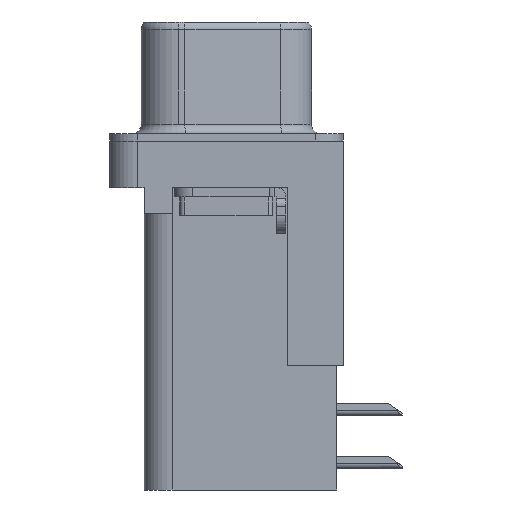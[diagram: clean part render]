
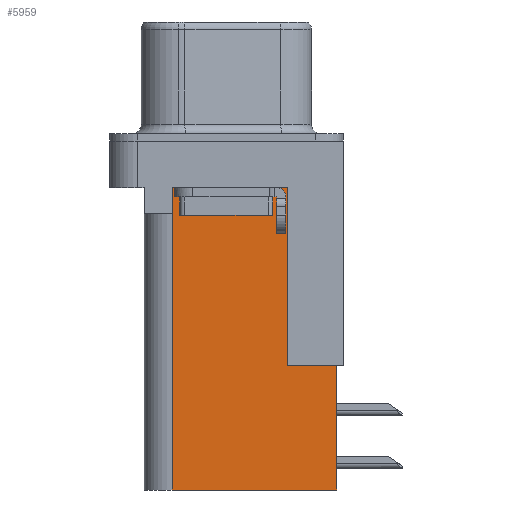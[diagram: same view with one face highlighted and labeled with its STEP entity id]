
A CAD part, left-side view. The second image highlights one B-rep face of the part: STEP entity #5959.
In plain terms, the highlighted planar face has unit normal (-1, 0, 0).
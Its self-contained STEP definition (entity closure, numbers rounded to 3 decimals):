
#126 = CARTESIAN_POINT ( 'NONE',  ( 3.765, -5.925, -2. ) ) ;
#256 = VECTOR ( 'NONE', #9642, 1000. ) ;
#456 = LINE ( 'NONE', #14605, #256 ) ;
#901 = CARTESIAN_POINT ( 'NONE',  ( 3.765, 2.895, -3.9 ) ) ;
#952 = VECTOR ( 'NONE', #4581, 1000. ) ;
#986 = DIRECTION ( 'NONE',  ( 0., 1., 0. ) ) ;
#1053 = LINE ( 'NONE', #12186, #952 ) ;
#1066 = CARTESIAN_POINT ( 'NONE',  ( 3.765, -6.295, -12.05 ) ) ;
#1239 = ORIENTED_EDGE ( 'NONE', *, *, #4993, .F. ) ;
#1700 = EDGE_LOOP ( 'NONE', ( #2459, #14002, #16082, #8216, #1239, #6621, #13790, #6805 ) ) ;
#1952 = LINE ( 'NONE', #14886, #2027 ) ;
#2027 = VECTOR ( 'NONE', #6052, 1000. ) ;
#2459 = ORIENTED_EDGE ( 'NONE', *, *, #7553, .T. ) ;
#2877 = EDGE_CURVE ( 'NONE', #8169, #6811, #7024, .T. ) ;
#3141 = DIRECTION ( 'NONE',  ( 1., 0., 0. ) ) ;
#3420 = CARTESIAN_POINT ( 'NONE',  ( 3.765, 2.925, -18.76 ) ) ;
#3614 = EDGE_CURVE ( 'NONE', #8169, #12137, #4800, .T. ) ;
#4581 = DIRECTION ( 'NONE',  ( 0., 1., 0. ) ) ;
#4800 = LINE ( 'NONE', #1066, #4847 ) ;
#4823 = CARTESIAN_POINT ( 'NONE',  ( 3.765, -3.295, -12.05 ) ) ;
#4847 = VECTOR ( 'NONE', #986, 1000. ) ;
#4993 = EDGE_CURVE ( 'NONE', #6811, #10145, #1053, .T. ) ;
#5348 = VECTOR ( 'NONE', #11344, 1000. ) ;
#5446 = LINE ( 'NONE', #901, #5348 ) ;
#5807 = DIRECTION ( 'NONE',  ( 0., 0., -1. ) ) ;
#5915 = VERTEX_POINT ( 'NONE', #12003 ) ;
#5959 = ADVANCED_FACE ( 'NONE', ( #14445 ), #8398, .F. ) ;
#6052 = DIRECTION ( 'NONE',  ( 0., 1., 0. ) ) ;
#6077 = VERTEX_POINT ( 'NONE', #8673 ) ;
#6144 = CARTESIAN_POINT ( 'NONE',  ( 3.765, -5.925, -12.05 ) ) ;
#6621 = ORIENTED_EDGE ( 'NONE', *, *, #2877, .F. ) ;
#6805 = ORIENTED_EDGE ( 'NONE', *, *, #13910, .T. ) ;
#6811 = VERTEX_POINT ( 'NONE', #9026 ) ;
#7024 = LINE ( 'NONE', #126, #7094 ) ;
#7047 = CARTESIAN_POINT ( 'NONE',  ( 3.765, -3.295, -18.76 ) ) ;
#7094 = VECTOR ( 'NONE', #5807, 1000. ) ;
#7225 = VECTOR ( 'NONE', #8335, 1000. ) ;
#7266 = LINE ( 'NONE', #14501, #7225 ) ;
#7553 = EDGE_CURVE ( 'NONE', #6077, #5915, #9296, .T. ) ;
#7623 = VERTEX_POINT ( 'NONE', #12732 ) ;
#7832 = CARTESIAN_POINT ( 'NONE',  ( 3.765, 2.925, -3.9 ) ) ;
#8169 = VERTEX_POINT ( 'NONE', #6144 ) ;
#8216 = ORIENTED_EDGE ( 'NONE', *, *, #15771, .F. ) ;
#8335 = DIRECTION ( 'NONE',  ( 0., 0., 1. ) ) ;
#8398 = PLANE ( 'NONE',  #14071 ) ;
#8673 = CARTESIAN_POINT ( 'NONE',  ( 3.765, -3.295, -2.5 ) ) ;
#8882 = EDGE_CURVE ( 'NONE', #5915, #7623, #5446, .T. ) ;
#8885 = CARTESIAN_POINT ( 'NONE',  ( 3.765, -3.295, -2.5 ) ) ;
#9026 = CARTESIAN_POINT ( 'NONE',  ( 3.765, -5.925, -18.76 ) ) ;
#9296 = LINE ( 'NONE', #8885, #9344 ) ;
#9344 = VECTOR ( 'NONE', #10108, 1000. ) ;
#9551 = VERTEX_POINT ( 'NONE', #7832 ) ;
#9642 = DIRECTION ( 'NONE',  ( 0., 0., 1. ) ) ;
#10108 = DIRECTION ( 'NONE',  ( 0., 1., 0. ) ) ;
#10145 = VERTEX_POINT ( 'NONE', #3420 ) ;
#10156 = EDGE_CURVE ( 'NONE', #7623, #9551, #1952, .T. ) ;
#11344 = DIRECTION ( 'NONE',  ( 0., 0., -1. ) ) ;
#12003 = CARTESIAN_POINT ( 'NONE',  ( 3.765, 2.895, -2.5 ) ) ;
#12101 = DIRECTION ( 'NONE',  ( 0., 1., 0. ) ) ;
#12137 = VERTEX_POINT ( 'NONE', #4823 ) ;
#12186 = CARTESIAN_POINT ( 'NONE',  ( 3.765, -3.295, -18.76 ) ) ;
#12732 = CARTESIAN_POINT ( 'NONE',  ( 3.765, 2.895, -3.9 ) ) ;
#13790 = ORIENTED_EDGE ( 'NONE', *, *, #3614, .T. ) ;
#13910 = EDGE_CURVE ( 'NONE', #12137, #6077, #7266, .T. ) ;
#14002 = ORIENTED_EDGE ( 'NONE', *, *, #8882, .T. ) ;
#14071 = AXIS2_PLACEMENT_3D ( 'NONE', #7047, #3141, #12101 ) ;
#14445 = FACE_OUTER_BOUND ( 'NONE', #1700, .T. ) ;
#14501 = CARTESIAN_POINT ( 'NONE',  ( 3.765, -3.295, -18.76 ) ) ;
#14605 = CARTESIAN_POINT ( 'NONE',  ( 3.765, 2.925, -18.76 ) ) ;
#14886 = CARTESIAN_POINT ( 'NONE',  ( 3.765, 0., -3.9 ) ) ;
#15771 = EDGE_CURVE ( 'NONE', #10145, #9551, #456, .T. ) ;
#16082 = ORIENTED_EDGE ( 'NONE', *, *, #10156, .T. ) ;
